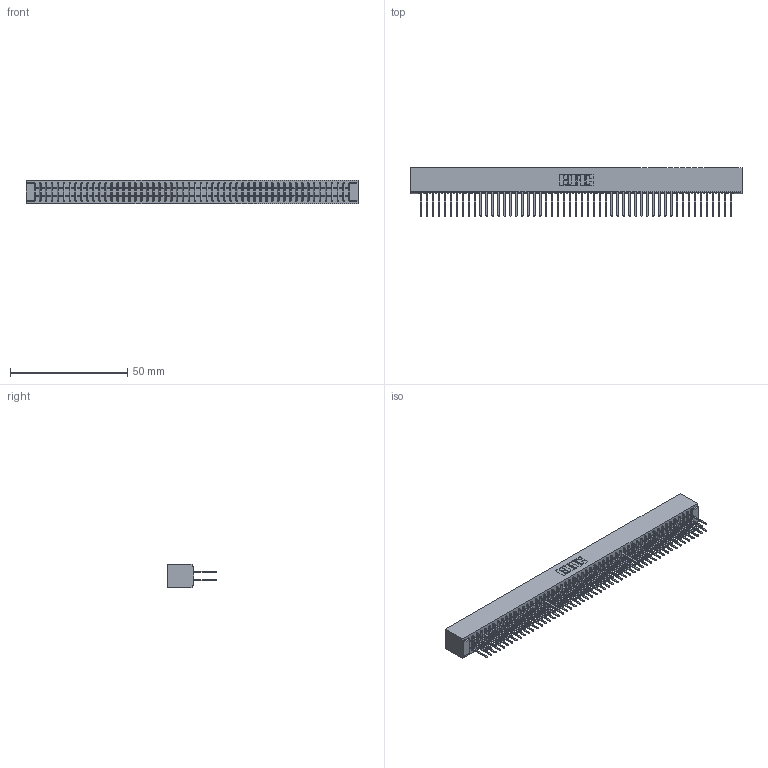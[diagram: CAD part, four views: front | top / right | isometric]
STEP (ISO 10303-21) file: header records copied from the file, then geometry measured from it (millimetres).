
FILE_DESCRIPTION (( 'STEP AP203' ), '1' );
FILE_NAME ('341-106-522-201.STEP', '2018-08-08T11:54:24', ( '' ), ( '' ), 'SwSTEP 2.0', 'SolidWorks 2016', '' );
FILE_SCHEMA (( 'CONFIG_CONTROL_DESIGN' ));
Length unit declared in the file: inch
Products named in the file (3): 341-292-001_341-292-122; 341 Part_No Mounting Lugs; 341-106-522-201
Assembly tree (107 placements, depth 2):
  341-106-522-201
    341 Part_No Mounting Lugs
    341-292-001_341-292-122  x106
Bounding box: 141.6 x 20.62 x 10.16 mm (x, y, z)
Volume: 10847.6 mm3; surface area: 21214.7 mm2
Topology: 107 solids, 107 shells, 7104 faces, 20591 edges, 13334 vertices
Faces by surface type: plane 4304, cylinder 2588, sphere 108, torus 104
Entity records: 62398 total; most frequent: CARTESIAN_POINT 10371, ORIENTED_EDGE 10306, DIRECTION 10055, EDGE_CURVE 5153, LINE 4179, VECTOR 4179, VERTEX_POINT 3254, AXIS2_PLACEMENT_3D 2938
